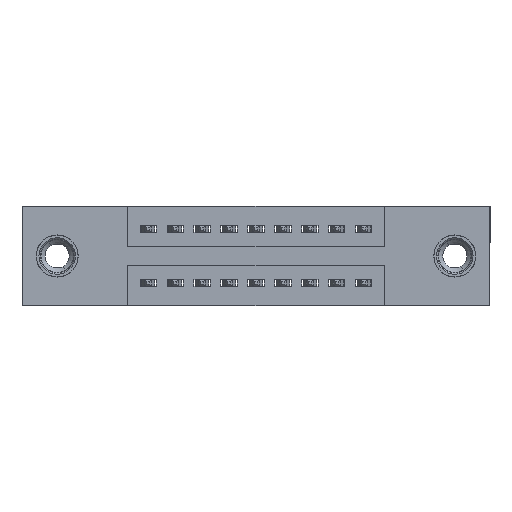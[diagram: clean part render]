
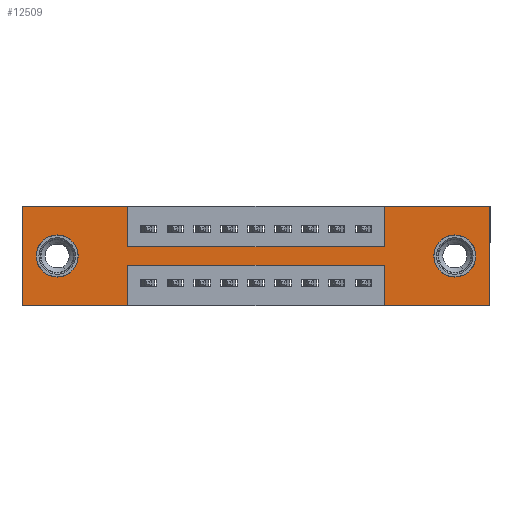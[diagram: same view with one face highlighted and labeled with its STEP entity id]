
A CAD part, front view. The second image highlights one B-rep face of the part: STEP entity #12509.
In plain terms, the highlighted planar face has unit normal (0, -1, 0).
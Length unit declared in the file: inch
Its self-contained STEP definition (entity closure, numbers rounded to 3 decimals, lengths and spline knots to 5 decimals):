
#133 = CARTESIAN_POINT ( 'NONE',  ( 0.13, 0., -0.185 ) ) ;
#229 = CARTESIAN_POINT ( 'NONE',  ( 1.605, 0., -0.185 ) ) ;
#350 = EDGE_CURVE ( 'NONE', #8833, #4774, #2054, .T. ) ;
#476 = CARTESIAN_POINT ( 'NONE',  ( 1.735, 0., -0.37 ) ) ;
#518 = FACE_BOUND ( 'NONE', #6160, .T. ) ;
#978 = LINE ( 'NONE', #14796, #7388 ) ;
#1062 = CARTESIAN_POINT ( 'NONE',  ( 0., 0., -0.37 ) ) ;
#1075 = ORIENTED_EDGE ( 'NONE', *, *, #7767, .F. ) ;
#1198 = CIRCLE ( 'NONE', #8895, 0.078 ) ;
#1412 = DIRECTION ( 'NONE',  ( 0., 0., 1. ) ) ;
#1429 = VERTEX_POINT ( 'NONE', #2304 ) ;
#1512 = DIRECTION ( 'NONE',  ( 0., 0., -1. ) ) ;
#1792 = CIRCLE ( 'NONE', #8404, 0.078 ) ;
#1803 = LINE ( 'NONE', #2550, #11529 ) ;
#1838 = VERTEX_POINT ( 'NONE', #9729 ) ;
#1852 = DIRECTION ( 'NONE',  ( 0., 0., 1. ) ) ;
#1895 = EDGE_CURVE ( 'NONE', #3877, #5653, #8379, .T. ) ;
#1908 = CARTESIAN_POINT ( 'NONE',  ( 0., 0., -0.37 ) ) ;
#2013 = CARTESIAN_POINT ( 'NONE',  ( 0., 0., -0.37 ) ) ;
#2054 = LINE ( 'NONE', #14868, #15832 ) ;
#2178 = CARTESIAN_POINT ( 'NONE',  ( 0., 0., 0. ) ) ;
#2292 = EDGE_CURVE ( 'NONE', #5010, #3877, #8984, .T. ) ;
#2304 = CARTESIAN_POINT ( 'NONE',  ( 1.3425, 0., 0. ) ) ;
#2440 = VECTOR ( 'NONE', #12315, 39.37008 ) ;
#2499 = ORIENTED_EDGE ( 'NONE', *, *, #11536, .F. ) ;
#2550 = CARTESIAN_POINT ( 'NONE',  ( 1.3425, 0., -0.37 ) ) ;
#2653 = AXIS2_PLACEMENT_3D ( 'NONE', #1908, #11996, #12046 ) ;
#2835 = EDGE_CURVE ( 'NONE', #1838, #8833, #1803, .T. ) ;
#2910 = CARTESIAN_POINT ( 'NONE',  ( 0.13, 0., -0.263 ) ) ;
#2915 = ORIENTED_EDGE ( 'NONE', *, *, #12656, .F. ) ;
#2985 = CARTESIAN_POINT ( 'NONE',  ( 0., 0., 0. ) ) ;
#3006 = DIRECTION ( 'NONE',  ( -1., 0., 0. ) ) ;
#3072 = LINE ( 'NONE', #9743, #5660 ) ;
#3114 = ORIENTED_EDGE ( 'NONE', *, *, #1895, .F. ) ;
#3190 = DIRECTION ( 'NONE',  ( 0., 0., -1. ) ) ;
#3193 = EDGE_LOOP ( 'NONE', ( #2915, #6317, #9637, #3321, #6713, #11047, #11989, #1075, #5288, #2499, #3114, #3225 ) ) ;
#3209 = PLANE ( 'NONE',  #2653 ) ;
#3225 = ORIENTED_EDGE ( 'NONE', *, *, #2292, .F. ) ;
#3245 = CARTESIAN_POINT ( 'NONE',  ( 1.605, 0., -0.263 ) ) ;
#3321 = ORIENTED_EDGE ( 'NONE', *, *, #9817, .F. ) ;
#3394 = LINE ( 'NONE', #9999, #10507 ) ;
#3612 = EDGE_CURVE ( 'NONE', #12063, #1429, #10898, .T. ) ;
#3614 = DIRECTION ( 'NONE',  ( -1., 0., 0. ) ) ;
#3668 = EDGE_CURVE ( 'NONE', #14012, #5525, #3394, .T. ) ;
#3673 = VERTEX_POINT ( 'NONE', #14411 ) ;
#3877 = VERTEX_POINT ( 'NONE', #1062 ) ;
#4184 = EDGE_CURVE ( 'NONE', #11836, #12266, #6370, .T. ) ;
#4220 = VECTOR ( 'NONE', #9392, 39.37008 ) ;
#4774 = VERTEX_POINT ( 'NONE', #7919 ) ;
#5010 = VERTEX_POINT ( 'NONE', #15851 ) ;
#5105 = ORIENTED_EDGE ( 'NONE', *, *, #14599, .T. ) ;
#5288 = ORIENTED_EDGE ( 'NONE', *, *, #14363, .F. ) ;
#5464 = DIRECTION ( 'NONE',  ( 0., 0., 1. ) ) ;
#5525 = VERTEX_POINT ( 'NONE', #476 ) ;
#5653 = VERTEX_POINT ( 'NONE', #14604 ) ;
#5658 = CARTESIAN_POINT ( 'NONE',  ( 1.605, 0., -0.185 ) ) ;
#5660 = VECTOR ( 'NONE', #14764, 39.37008 ) ;
#5802 = CARTESIAN_POINT ( 'NONE',  ( 0.13, 0., -0.185 ) ) ;
#6063 = CARTESIAN_POINT ( 'NONE',  ( 0.3925, 0., 0. ) ) ;
#6160 = EDGE_LOOP ( 'NONE', ( #11423, #5105 ) ) ;
#6317 = ORIENTED_EDGE ( 'NONE', *, *, #350, .F. ) ;
#6370 = CIRCLE ( 'NONE', #9139, 0.078 ) ;
#6713 = ORIENTED_EDGE ( 'NONE', *, *, #3668, .F. ) ;
#6762 = CARTESIAN_POINT ( 'NONE',  ( 1.3425, 0., -0.22 ) ) ;
#6940 = DIRECTION ( 'NONE',  ( 0., 0., -1. ) ) ;
#7085 = DIRECTION ( 'NONE',  ( 0., 0., 1. ) ) ;
#7287 = VERTEX_POINT ( 'NONE', #12458 ) ;
#7388 = VECTOR ( 'NONE', #16012, 39.37008 ) ;
#7436 = AXIS2_PLACEMENT_3D ( 'NONE', #5802, #14558, #7085 ) ;
#7767 = EDGE_CURVE ( 'NONE', #3673, #12063, #3072, .T. ) ;
#7919 = CARTESIAN_POINT ( 'NONE',  ( 0.3925, 0., -0.22 ) ) ;
#7991 = VECTOR ( 'NONE', #13602, 39.37008 ) ;
#8157 = CIRCLE ( 'NONE', #7436, 0.078 ) ;
#8289 = LINE ( 'NONE', #11044, #14544 ) ;
#8379 = LINE ( 'NONE', #2985, #4220 ) ;
#8404 = AXIS2_PLACEMENT_3D ( 'NONE', #229, #9105, #1512 ) ;
#8481 = EDGE_CURVE ( 'NONE', #1429, #14012, #12520, .T. ) ;
#8833 = VERTEX_POINT ( 'NONE', #6762 ) ;
#8868 = ORIENTED_EDGE ( 'NONE', *, *, #10228, .T. ) ;
#8895 = AXIS2_PLACEMENT_3D ( 'NONE', #5658, #14428, #6940 ) ;
#8984 = LINE ( 'NONE', #2013, #15225 ) ;
#9024 = DIRECTION ( 'NONE',  ( 0., 1., 0. ) ) ;
#9105 = DIRECTION ( 'NONE',  ( 0., 1., 0. ) ) ;
#9126 = CARTESIAN_POINT ( 'NONE',  ( 1.605, 0., -0.107 ) ) ;
#9139 = AXIS2_PLACEMENT_3D ( 'NONE', #133, #9024, #1412 ) ;
#9280 = CARTESIAN_POINT ( 'NONE',  ( 1.735, 0., 0. ) ) ;
#9392 = DIRECTION ( 'NONE',  ( 0., 0., 1. ) ) ;
#9546 = EDGE_CURVE ( 'NONE', #14985, #12000, #1198, .T. ) ;
#9637 = ORIENTED_EDGE ( 'NONE', *, *, #2835, .F. ) ;
#9729 = CARTESIAN_POINT ( 'NONE',  ( 1.3425, 0., -0.37 ) ) ;
#9743 = CARTESIAN_POINT ( 'NONE',  ( 0.3925, 0., -0.15 ) ) ;
#9817 = EDGE_CURVE ( 'NONE', #5525, #1838, #978, .T. ) ;
#9999 = CARTESIAN_POINT ( 'NONE',  ( 1.735, 0., 0. ) ) ;
#10228 = EDGE_CURVE ( 'NONE', #12266, #11836, #8157, .T. ) ;
#10507 = VECTOR ( 'NONE', #3190, 39.37008 ) ;
#10898 = LINE ( 'NONE', #13823, #13813 ) ;
#11044 = CARTESIAN_POINT ( 'NONE',  ( 0.3925, 0., -0.37 ) ) ;
#11047 = ORIENTED_EDGE ( 'NONE', *, *, #8481, .F. ) ;
#11328 = LINE ( 'NONE', #6063, #7991 ) ;
#11423 = ORIENTED_EDGE ( 'NONE', *, *, #9546, .T. ) ;
#11529 = VECTOR ( 'NONE', #1852, 39.37008 ) ;
#11536 = EDGE_CURVE ( 'NONE', #5653, #7287, #13603, .T. ) ;
#11836 = VERTEX_POINT ( 'NONE', #2910 ) ;
#11989 = ORIENTED_EDGE ( 'NONE', *, *, #3612, .F. ) ;
#11996 = DIRECTION ( 'NONE',  ( 0., -1., 0. ) ) ;
#12000 = VERTEX_POINT ( 'NONE', #3245 ) ;
#12046 = DIRECTION ( 'NONE',  ( 0., 0., -1. ) ) ;
#12063 = VERTEX_POINT ( 'NONE', #14673 ) ;
#12199 = ORIENTED_EDGE ( 'NONE', *, *, #4184, .T. ) ;
#12266 = VERTEX_POINT ( 'NONE', #12615 ) ;
#12313 = DIRECTION ( 'NONE',  ( 0., 0., -1. ) ) ;
#12315 = DIRECTION ( 'NONE',  ( 1., 0., 0. ) ) ;
#12458 = CARTESIAN_POINT ( 'NONE',  ( 0.3925, 0., 0. ) ) ;
#12509 = ADVANCED_FACE ( 'NONE', ( #518, #13962, #13184 ), #3209, .T. ) ;
#12520 = LINE ( 'NONE', #2178, #2440 ) ;
#12615 = CARTESIAN_POINT ( 'NONE',  ( 0.13, 0., -0.107 ) ) ;
#12656 = EDGE_CURVE ( 'NONE', #4774, #5010, #8289, .T. ) ;
#13134 = EDGE_LOOP ( 'NONE', ( #8868, #12199 ) ) ;
#13184 = FACE_OUTER_BOUND ( 'NONE', #3193, .T. ) ;
#13216 = VECTOR ( 'NONE', #15864, 39.37008 ) ;
#13602 = DIRECTION ( 'NONE',  ( 0., 0., -1. ) ) ;
#13603 = LINE ( 'NONE', #14636, #13216 ) ;
#13813 = VECTOR ( 'NONE', #5464, 39.37008 ) ;
#13823 = CARTESIAN_POINT ( 'NONE',  ( 1.3425, 0., 0. ) ) ;
#13962 = FACE_BOUND ( 'NONE', #13134, .T. ) ;
#14012 = VERTEX_POINT ( 'NONE', #9280 ) ;
#14363 = EDGE_CURVE ( 'NONE', #7287, #3673, #11328, .T. ) ;
#14411 = CARTESIAN_POINT ( 'NONE',  ( 0.3925, 0., -0.15 ) ) ;
#14428 = DIRECTION ( 'NONE',  ( 0., 1., 0. ) ) ;
#14544 = VECTOR ( 'NONE', #12313, 39.37008 ) ;
#14558 = DIRECTION ( 'NONE',  ( 0., 1., 0. ) ) ;
#14599 = EDGE_CURVE ( 'NONE', #12000, #14985, #1792, .T. ) ;
#14604 = CARTESIAN_POINT ( 'NONE',  ( 0., 0., 0. ) ) ;
#14636 = CARTESIAN_POINT ( 'NONE',  ( 0., 0., 0. ) ) ;
#14673 = CARTESIAN_POINT ( 'NONE',  ( 1.3425, 0., -0.15 ) ) ;
#14764 = DIRECTION ( 'NONE',  ( 1., 0., 0. ) ) ;
#14796 = CARTESIAN_POINT ( 'NONE',  ( 0., 0., -0.37 ) ) ;
#14868 = CARTESIAN_POINT ( 'NONE',  ( 0.3925, 0., -0.22 ) ) ;
#14985 = VERTEX_POINT ( 'NONE', #9126 ) ;
#15225 = VECTOR ( 'NONE', #3006, 39.37008 ) ;
#15832 = VECTOR ( 'NONE', #3614, 39.37008 ) ;
#15851 = CARTESIAN_POINT ( 'NONE',  ( 0.3925, 0., -0.37 ) ) ;
#15864 = DIRECTION ( 'NONE',  ( 1., 0., 0. ) ) ;
#16012 = DIRECTION ( 'NONE',  ( -1., 0., 0. ) ) ;
